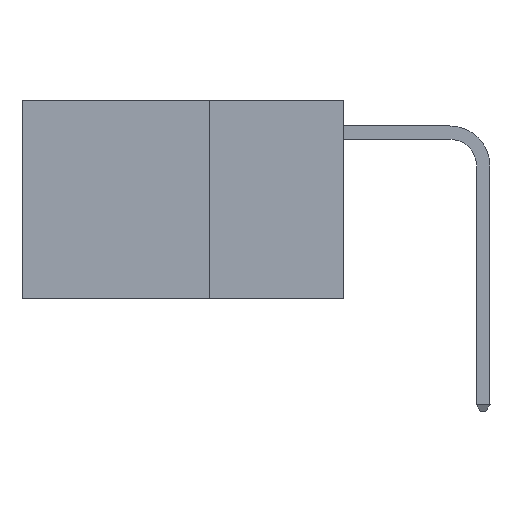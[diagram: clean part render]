
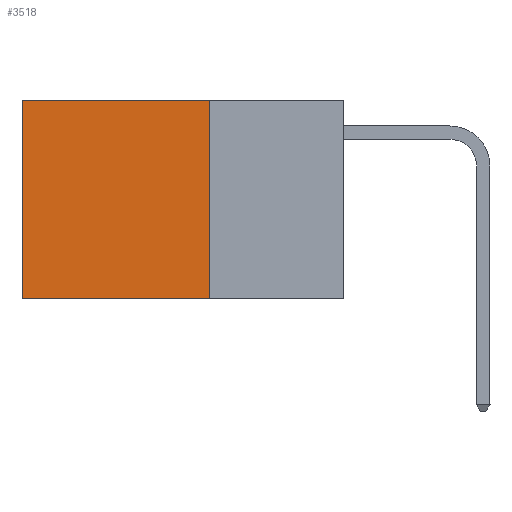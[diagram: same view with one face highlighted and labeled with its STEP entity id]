
A CAD part, left-side view. The second image highlights one B-rep face of the part: STEP entity #3518.
In plain terms, the highlighted planar face has unit normal (-1, 0, 0).
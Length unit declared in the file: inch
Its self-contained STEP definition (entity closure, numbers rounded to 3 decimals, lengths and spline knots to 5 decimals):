
#233 = VERTEX_POINT ( 'NONE', #15361 ) ;
#2160 = EDGE_CURVE ( 'NONE', #14379, #233, #4266, .T. ) ;
#2694 = VERTEX_POINT ( 'NONE', #10455 ) ;
#3518 = ADVANCED_FACE ( 'NONE', ( #20173 ), #15054, .F. ) ;
#3790 = ORIENTED_EDGE ( 'NONE', *, *, #2160, .T. ) ;
#4266 = LINE ( 'NONE', #22697, #21886 ) ;
#6373 = DIRECTION ( 'NONE',  ( 1., 0., 0. ) ) ;
#6538 = LINE ( 'NONE', #22589, #8204 ) ;
#6748 = LINE ( 'NONE', #11190, #22439 ) ;
#7058 = EDGE_CURVE ( 'NONE', #2694, #14379, #6538, .T. ) ;
#7423 = VECTOR ( 'NONE', #25298, 39.37008 ) ;
#7594 = CARTESIAN_POINT ( 'NONE',  ( 0.2625, 0.25, 0. ) ) ;
#7647 = CARTESIAN_POINT ( 'NONE',  ( 0.2625, 0.6, 0. ) ) ;
#8204 = VECTOR ( 'NONE', #15806, 39.37008 ) ;
#8210 = ORIENTED_EDGE ( 'NONE', *, *, #11397, .F. ) ;
#10455 = CARTESIAN_POINT ( 'NONE',  ( 0.2625, 0.25, 0. ) ) ;
#11037 = EDGE_CURVE ( 'NONE', #11093, #233, #6748, .T. ) ;
#11093 = VERTEX_POINT ( 'NONE', #21248 ) ;
#11190 = CARTESIAN_POINT ( 'NONE',  ( 0.2625, 0.25, -0.37 ) ) ;
#11397 = EDGE_CURVE ( 'NONE', #2694, #11093, #25447, .T. ) ;
#11695 = EDGE_LOOP ( 'NONE', ( #3790, #15700, #8210, #24387 ) ) ;
#14379 = VERTEX_POINT ( 'NONE', #7647 ) ;
#15054 = PLANE ( 'NONE',  #18519 ) ;
#15361 = CARTESIAN_POINT ( 'NONE',  ( 0.2625, 0.6, -0.37 ) ) ;
#15640 = DIRECTION ( 'NONE',  ( 0., 0., -1. ) ) ;
#15700 = ORIENTED_EDGE ( 'NONE', *, *, #11037, .F. ) ;
#15806 = DIRECTION ( 'NONE',  ( 0., 1., 0. ) ) ;
#18519 = AXIS2_PLACEMENT_3D ( 'NONE', #27116, #6373, #15640 ) ;
#20173 = FACE_OUTER_BOUND ( 'NONE', #11695, .T. ) ;
#21248 = CARTESIAN_POINT ( 'NONE',  ( 0.2625, 0.25, -0.37 ) ) ;
#21886 = VECTOR ( 'NONE', #27393, 39.37008 ) ;
#22439 = VECTOR ( 'NONE', #29650, 39.37008 ) ;
#22589 = CARTESIAN_POINT ( 'NONE',  ( 0.2625, 0.25, 0. ) ) ;
#22697 = CARTESIAN_POINT ( 'NONE',  ( 0.2625, 0.6, 0. ) ) ;
#24387 = ORIENTED_EDGE ( 'NONE', *, *, #7058, .T. ) ;
#25298 = DIRECTION ( 'NONE',  ( 0., 0., -1. ) ) ;
#25447 = LINE ( 'NONE', #7594, #7423 ) ;
#27116 = CARTESIAN_POINT ( 'NONE',  ( 0.2625, 0.25, 0. ) ) ;
#27393 = DIRECTION ( 'NONE',  ( 0., 0., -1. ) ) ;
#29650 = DIRECTION ( 'NONE',  ( 0., 1., 0. ) ) ;
